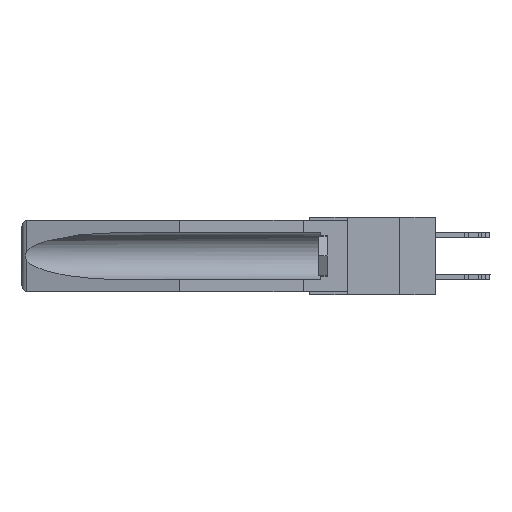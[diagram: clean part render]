
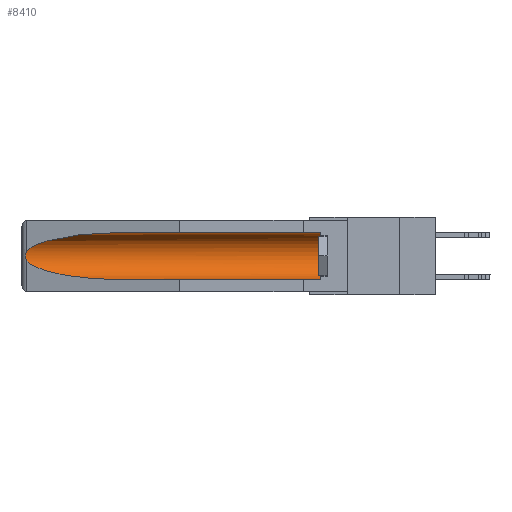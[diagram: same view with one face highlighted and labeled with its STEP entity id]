
A CAD part, left-side view. The second image highlights one B-rep face of the part: STEP entity #8410.
In plain terms, the highlighted cylindrical face has radius 2.857 mm (diameter 5.715 mm), a partial arc.
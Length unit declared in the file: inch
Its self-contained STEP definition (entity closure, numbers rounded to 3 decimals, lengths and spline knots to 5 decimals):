
#412 = CARTESIAN_POINT ( 'NONE',  ( 0.26537, 1.52718, -0.14972 ) ) ;
#946 = CARTESIAN_POINT ( 'NONE',  ( 0.26655, 1.53094, -0.18657 ) ) ;
#1391 = ORIENTED_EDGE ( 'NONE', *, *, #4666, .T. ) ;
#1764 = EDGE_CURVE ( 'NONE', #24947, #9979, #21963, .T. ) ;
#2760 = CARTESIAN_POINT ( 'NONE',  ( 0.26597, 1.52961, -0.15275 ) ) ;
#2956 = CARTESIAN_POINT ( 'NONE',  ( 0.155, 0.126, -0.1715 ) ) ;
#4053 = CARTESIAN_POINT ( 'NONE',  ( 0.155, -0.30754, -0.059 ) ) ;
#4666 = EDGE_CURVE ( 'NONE', #7385, #24947, #6835, .T. ) ;
#5350 = ORIENTED_EDGE ( 'NONE', *, *, #8799, .T. ) ;
#6234 = VECTOR ( 'NONE', #27486, 39.37008 ) ;
#6835 = B_SPLINE_CURVE_WITH_KNOTS ( 'NONE', 3,
 ( #412, #2760, #19268, #8849, #22342, #22861, #12807, #946, #22155, #24523 ),
 .UNSPECIFIED., .F., .F.,
 ( 4, 2, 2, 2, 4 ),
 ( 0., 0.00029, 0.00058, 0.00087, 0.00117 ),
 .UNSPECIFIED. ) ;
#7385 = VERTEX_POINT ( 'NONE', #22499 ) ;
#7598 = VECTOR ( 'NONE', #20564, 39.37008 ) ;
#8095 = CARTESIAN_POINT ( 'NONE',  ( 0.21114, 1.30732, -0.284 ) ) ;
#8410 = ADVANCED_FACE ( 'NONE', ( #26455 ), #20902, .F. ) ;
#8554 = VERTEX_POINT ( 'NONE', #27490 ) ;
#8799 = EDGE_CURVE ( 'NONE', #17829, #20882, #30143, .T. ) ;
#8849 = CARTESIAN_POINT ( 'NONE',  ( 0.2673, 1.5327, -0.16383 ) ) ;
#9067 = CARTESIAN_POINT ( 'NONE',  ( 0.21114, 1.30732, -0.059 ) ) ;
#9979 = VERTEX_POINT ( 'NONE', #22817 ) ;
#10650 = CIRCLE ( 'NONE', #20024, 0.1125 ) ;
#12156 = ORIENTED_EDGE ( 'NONE', *, *, #28374, .F. ) ;
#12577 = AXIS2_PLACEMENT_3D ( 'NONE', #20956, #28302, #16136 ) ;
#12807 = CARTESIAN_POINT ( 'NONE',  ( 0.2673, 1.53269, -0.17917 ) ) ;
#13200 = CARTESIAN_POINT ( 'NONE',  ( 0.26537, 1.52718, -0.14972 ) ) ;
#14954 = EDGE_CURVE ( 'NONE', #8554, #17829, #10650, .T. ) ;
#15019 = DIRECTION ( 'NONE',  ( 0., 0., 1. ) ) ;
#15229 = CARTESIAN_POINT ( 'NONE',  ( 0.25451, 1.48313, -0.24835 ) ) ;
#15376 = CARTESIAN_POINT ( 'NONE',  ( 0.155, 1.07973, -0.059 ) ) ;
#15711 = CARTESIAN_POINT ( 'NONE',  ( 0.155, 0.126, -0.059 ) ) ;
#15817 = EDGE_CURVE ( 'NONE', #20882, #7385, #30309, .T. ) ;
#16019 = CARTESIAN_POINT ( 'NONE',  ( 0.155, -0.30754, -0.284 ) ) ;
#16112 = CARTESIAN_POINT ( 'NONE',  ( 0.25451, 1.48313, -0.09465 ) ) ;
#16136 = DIRECTION ( 'NONE',  ( 0., 0., 1. ) ) ;
#16183 = CARTESIAN_POINT ( 'NONE',  ( 0.155, 1.07973, -0.059 ) ) ;
#17829 = VERTEX_POINT ( 'NONE', #15711 ) ;
#19268 = CARTESIAN_POINT ( 'NONE',  ( 0.26654, 1.53092, -0.15636 ) ) ;
#20024 = AXIS2_PLACEMENT_3D ( 'NONE', #2956, #29161, #15019 ) ;
#20263 = CARTESIAN_POINT ( 'NONE',  ( 0.26537, 1.52718, -0.19328 ) ) ;
#20564 = DIRECTION ( 'NONE',  ( 0., 1., 0. ) ) ;
#20882 = VERTEX_POINT ( 'NONE', #16183 ) ;
#20902 = CYLINDRICAL_SURFACE ( 'NONE', #12577, 0.1125 ) ;
#20956 = CARTESIAN_POINT ( 'NONE',  ( 0.155, -0.30754, -0.1715 ) ) ;
#21963 =( BOUNDED_CURVE ( )  B_SPLINE_CURVE ( 3, ( #20263, #15229, #8095, #22238 ),
 .UNSPECIFIED., .F., .F. ) 
 B_SPLINE_CURVE_WITH_KNOTS ( ( 4, 4 ),
 ( 0.1948, 1.5708 ),
 .UNSPECIFIED. ) 
 CURVE ( )  GEOMETRIC_REPRESENTATION_ITEM ( )  RATIONAL_B_SPLINE_CURVE ( ( 1., 0.848, 0.848, 1. ) ) 
 REPRESENTATION_ITEM ( '' )  );
#22155 = CARTESIAN_POINT ( 'NONE',  ( 0.26597, 1.5296, -0.19026 ) ) ;
#22238 = CARTESIAN_POINT ( 'NONE',  ( 0.155, 1.07973, -0.284 ) ) ;
#22342 = CARTESIAN_POINT ( 'NONE',  ( 0.2675, 1.53308, -0.16763 ) ) ;
#22499 = CARTESIAN_POINT ( 'NONE',  ( 0.26537, 1.52718, -0.14972 ) ) ;
#22817 = CARTESIAN_POINT ( 'NONE',  ( 0.155, 1.07973, -0.284 ) ) ;
#22861 = CARTESIAN_POINT ( 'NONE',  ( 0.2675, 1.53308, -0.17534 ) ) ;
#24523 = CARTESIAN_POINT ( 'NONE',  ( 0.26537, 1.52718, -0.19328 ) ) ;
#24947 = VERTEX_POINT ( 'NONE', #30545 ) ;
#26455 = FACE_OUTER_BOUND ( 'NONE', #29885, .T. ) ;
#27486 = DIRECTION ( 'NONE',  ( 0., 1., 0. ) ) ;
#27490 = CARTESIAN_POINT ( 'NONE',  ( 0.155, 0.126, -0.284 ) ) ;
#28035 = LINE ( 'NONE', #16019, #6234 ) ;
#28302 = DIRECTION ( 'NONE',  ( 0., 1., 0. ) ) ;
#28374 = EDGE_CURVE ( 'NONE', #8554, #9979, #28035, .T. ) ;
#28862 = ORIENTED_EDGE ( 'NONE', *, *, #1764, .T. ) ;
#29161 = DIRECTION ( 'NONE',  ( 0., -1., 0. ) ) ;
#29728 = ORIENTED_EDGE ( 'NONE', *, *, #14954, .T. ) ;
#29885 = EDGE_LOOP ( 'NONE', ( #30004, #1391, #28862, #12156, #29728, #5350 ) ) ;
#30004 = ORIENTED_EDGE ( 'NONE', *, *, #15817, .T. ) ;
#30143 = LINE ( 'NONE', #4053, #7598 ) ;
#30309 =( BOUNDED_CURVE ( )  B_SPLINE_CURVE ( 3, ( #15376, #9067, #16112, #13200 ),
 .UNSPECIFIED., .F., .F. ) 
 B_SPLINE_CURVE_WITH_KNOTS ( ( 4, 4 ),
 ( 4.71239, 6.08839 ),
 .UNSPECIFIED. ) 
 CURVE ( )  GEOMETRIC_REPRESENTATION_ITEM ( )  RATIONAL_B_SPLINE_CURVE ( ( 1., 0.848, 0.848, 1. ) ) 
 REPRESENTATION_ITEM ( '' )  );
#30545 = CARTESIAN_POINT ( 'NONE',  ( 0.26537, 1.52718, -0.19328 ) ) ;
